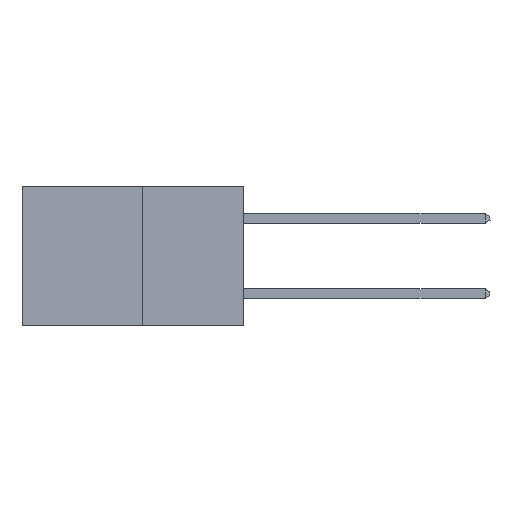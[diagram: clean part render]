
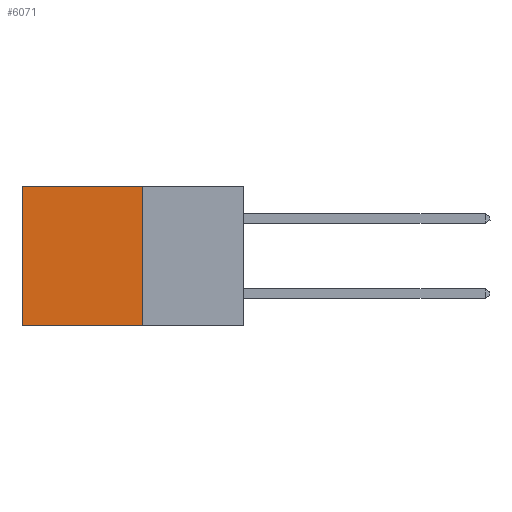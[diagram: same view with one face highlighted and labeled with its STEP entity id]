
A CAD part, left-side view. The second image highlights one B-rep face of the part: STEP entity #6071.
In plain terms, the highlighted planar face has unit normal (-1, 0, 0).
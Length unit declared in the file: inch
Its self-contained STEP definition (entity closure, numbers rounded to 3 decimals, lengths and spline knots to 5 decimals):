
#252 = LINE ( 'NONE', #987, #8279 ) ;
#472 = VECTOR ( 'NONE', #11796, 39.37008 ) ;
#987 = CARTESIAN_POINT ( 'NONE',  ( 0.277, 0.27, 0. ) ) ;
#1128 = CARTESIAN_POINT ( 'NONE',  ( 0.277, 0.27, 0. ) ) ;
#1380 = VERTEX_POINT ( 'NONE', #9577 ) ;
#1964 = EDGE_CURVE ( 'NONE', #9494, #1380, #252, .T. ) ;
#2911 = ORIENTED_EDGE ( 'NONE', *, *, #8240, .T. ) ;
#2942 = DIRECTION ( 'NONE',  ( 1., 0., 0. ) ) ;
#2969 = CARTESIAN_POINT ( 'NONE',  ( 0.277, 0.27, -0.37 ) ) ;
#3050 = VERTEX_POINT ( 'NONE', #8337 ) ;
#3191 = PLANE ( 'NONE',  #6791 ) ;
#3194 = LINE ( 'NONE', #3234, #11150 ) ;
#3234 = CARTESIAN_POINT ( 'NONE',  ( 0.277, 0.27, -0.37 ) ) ;
#3838 = CARTESIAN_POINT ( 'NONE',  ( 0.277, 0.27, -0.37 ) ) ;
#4127 = FACE_OUTER_BOUND ( 'NONE', #5943, .T. ) ;
#4296 = VECTOR ( 'NONE', #7291, 39.37008 ) ;
#5149 = EDGE_CURVE ( 'NONE', #6845, #3050, #3194, .T. ) ;
#5400 = LINE ( 'NONE', #11810, #472 ) ;
#5943 = EDGE_LOOP ( 'NONE', ( #2911, #8309, #6889, #11430 ) ) ;
#6071 = ADVANCED_FACE ( 'NONE', ( #4127 ), #3191, .F. ) ;
#6791 = AXIS2_PLACEMENT_3D ( 'NONE', #2969, #2942, #8010 ) ;
#6845 = VERTEX_POINT ( 'NONE', #3838 ) ;
#6889 = ORIENTED_EDGE ( 'NONE', *, *, #7172, .F. ) ;
#7172 = EDGE_CURVE ( 'NONE', #9494, #6845, #5400, .T. ) ;
#7251 = DIRECTION ( 'NONE',  ( 0., 1., 0. ) ) ;
#7291 = DIRECTION ( 'NONE',  ( 0., 0., -1. ) ) ;
#7317 = CARTESIAN_POINT ( 'NONE',  ( 0.277, 0.59, -0.37 ) ) ;
#8010 = DIRECTION ( 'NONE',  ( 0., 0., -1. ) ) ;
#8240 = EDGE_CURVE ( 'NONE', #1380, #3050, #11557, .T. ) ;
#8279 = VECTOR ( 'NONE', #8453, 39.37008 ) ;
#8309 = ORIENTED_EDGE ( 'NONE', *, *, #5149, .F. ) ;
#8337 = CARTESIAN_POINT ( 'NONE',  ( 0.277, 0.59, -0.37 ) ) ;
#8453 = DIRECTION ( 'NONE',  ( 0., 1., 0. ) ) ;
#9494 = VERTEX_POINT ( 'NONE', #1128 ) ;
#9577 = CARTESIAN_POINT ( 'NONE',  ( 0.277, 0.59, 0. ) ) ;
#11150 = VECTOR ( 'NONE', #7251, 39.37008 ) ;
#11430 = ORIENTED_EDGE ( 'NONE', *, *, #1964, .T. ) ;
#11557 = LINE ( 'NONE', #7317, #4296 ) ;
#11796 = DIRECTION ( 'NONE',  ( 0., 0., -1. ) ) ;
#11810 = CARTESIAN_POINT ( 'NONE',  ( 0.277, 0.27, -0.37 ) ) ;
